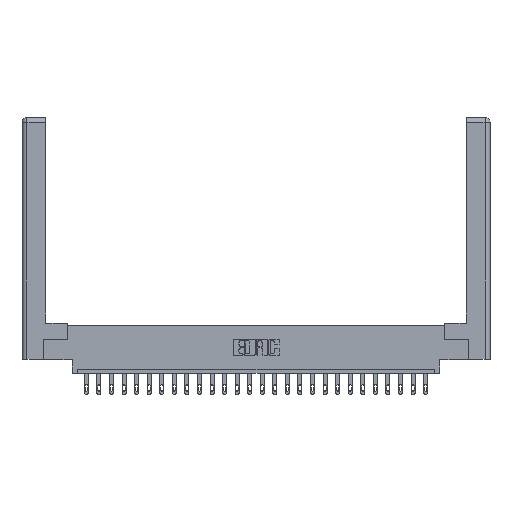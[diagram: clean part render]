
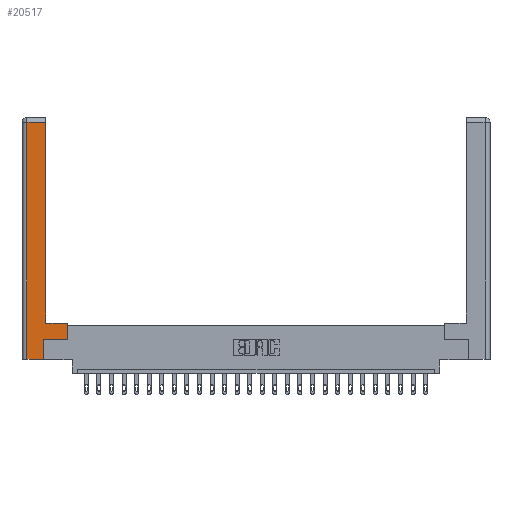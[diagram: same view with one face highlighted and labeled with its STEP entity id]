
A CAD part, top view. The second image highlights one B-rep face of the part: STEP entity #20517.
In plain terms, the highlighted planar face has unit normal (0, 0, 1).
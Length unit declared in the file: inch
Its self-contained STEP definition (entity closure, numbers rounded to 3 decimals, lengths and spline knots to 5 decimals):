
#212 = DIRECTION ( 'NONE',  ( 0., 1., 0. ) ) ;
#317 = VECTOR ( 'NONE', #12302, 39.37008 ) ;
#803 = CARTESIAN_POINT ( 'NONE',  ( 0.0615, 2.94, 0. ) ) ;
#1140 = CARTESIAN_POINT ( 'NONE',  ( 0.0615, 0., 0. ) ) ;
#1840 = CARTESIAN_POINT ( 'NONE',  ( 0.565, 0.245, 0. ) ) ;
#2126 = DIRECTION ( 'NONE',  ( -1., 0., 0. ) ) ;
#2163 = CARTESIAN_POINT ( 'NONE',  ( 0.295, 2.94, 0. ) ) ;
#2309 = ORIENTED_EDGE ( 'NONE', *, *, #22836, .T. ) ;
#2355 = CARTESIAN_POINT ( 'NONE',  ( 0.295, 0.45, 0. ) ) ;
#2630 = VECTOR ( 'NONE', #5573, 39.37008 ) ;
#3121 = ORIENTED_EDGE ( 'NONE', *, *, #6932, .T. ) ;
#3186 = ORIENTED_EDGE ( 'NONE', *, *, #24485, .T. ) ;
#3775 = CARTESIAN_POINT ( 'NONE',  ( 0.0615, 2.94, 0. ) ) ;
#4020 = ORIENTED_EDGE ( 'NONE', *, *, #15495, .T. ) ;
#4093 = VERTEX_POINT ( 'NONE', #1840 ) ;
#4378 = CARTESIAN_POINT ( 'NONE',  ( 0.295, 0.45, 0. ) ) ;
#4829 = VERTEX_POINT ( 'NONE', #2163 ) ;
#4913 = EDGE_CURVE ( 'NONE', #11134, #15058, #12675, .T. ) ;
#5312 = EDGE_CURVE ( 'NONE', #4093, #13347, #23640, .T. ) ;
#5573 = DIRECTION ( 'NONE',  ( 1., 0., 0. ) ) ;
#5865 = AXIS2_PLACEMENT_3D ( 'NONE', #18293, #6524, #23689 ) ;
#5906 = VECTOR ( 'NONE', #212, 39.37008 ) ;
#6524 = DIRECTION ( 'NONE',  ( 0., 0., -1. ) ) ;
#6556 = VECTOR ( 'NONE', #11963, 39.37008 ) ;
#6768 = VECTOR ( 'NONE', #14178, 39.37008 ) ;
#6932 = EDGE_CURVE ( 'NONE', #7507, #4093, #24185, .T. ) ;
#7394 = ORIENTED_EDGE ( 'NONE', *, *, #7652, .T. ) ;
#7507 = VERTEX_POINT ( 'NONE', #17565 ) ;
#7652 = EDGE_CURVE ( 'NONE', #17378, #7507, #19934, .T. ) ;
#7680 = VECTOR ( 'NONE', #2126, 39.37008 ) ;
#7844 = CARTESIAN_POINT ( 'NONE',  ( 0.0615, 0., 0. ) ) ;
#7941 = ORIENTED_EDGE ( 'NONE', *, *, #5312, .T. ) ;
#9828 = CARTESIAN_POINT ( 'NONE',  ( 0.295, 3., 0. ) ) ;
#11134 = VERTEX_POINT ( 'NONE', #803 ) ;
#11750 = LINE ( 'NONE', #2355, #6556 ) ;
#11867 = FACE_OUTER_BOUND ( 'NONE', #20392, .T. ) ;
#11963 = DIRECTION ( 'NONE',  ( -1., 0., 0. ) ) ;
#11996 = ORIENTED_EDGE ( 'NONE', *, *, #21440, .T. ) ;
#12302 = DIRECTION ( 'NONE',  ( 0., 1., 0. ) ) ;
#12675 = LINE ( 'NONE', #1140, #19402 ) ;
#12899 = LINE ( 'NONE', #3775, #7680 ) ;
#13347 = VERTEX_POINT ( 'NONE', #19667 ) ;
#14178 = DIRECTION ( 'NONE',  ( 1., 0., 0. ) ) ;
#14188 = PLANE ( 'NONE',  #5865 ) ;
#15058 = VERTEX_POINT ( 'NONE', #7844 ) ;
#15195 = VERTEX_POINT ( 'NONE', #4378 ) ;
#15319 = CARTESIAN_POINT ( 'NONE',  ( 0.265, 0., 0. ) ) ;
#15495 = EDGE_CURVE ( 'NONE', #13347, #15195, #11750, .T. ) ;
#15695 = CARTESIAN_POINT ( 'NONE',  ( 0.565, 0.245, 0. ) ) ;
#16761 = CARTESIAN_POINT ( 'NONE',  ( 0.265, 0., 0. ) ) ;
#17378 = VERTEX_POINT ( 'NONE', #15319 ) ;
#17565 = CARTESIAN_POINT ( 'NONE',  ( 0.265, 0.245, 0. ) ) ;
#18293 = CARTESIAN_POINT ( 'NONE',  ( 0., 0., 0. ) ) ;
#19402 = VECTOR ( 'NONE', #24981, 39.37008 ) ;
#19667 = CARTESIAN_POINT ( 'NONE',  ( 0.565, 0.45, 0. ) ) ;
#19934 = LINE ( 'NONE', #20092, #317 ) ;
#20038 = LINE ( 'NONE', #9828, #5906 ) ;
#20092 = CARTESIAN_POINT ( 'NONE',  ( 0.265, 0.245, 0. ) ) ;
#20392 = EDGE_LOOP ( 'NONE', ( #2309, #3186, #23152, #11996, #7394, #3121, #7941, #4020 ) ) ;
#20517 = ADVANCED_FACE ( 'NONE', ( #11867 ), #14188, .F. ) ;
#20714 = LINE ( 'NONE', #16761, #2630 ) ;
#20934 = VECTOR ( 'NONE', #24129, 39.37008 ) ;
#21440 = EDGE_CURVE ( 'NONE', #15058, #17378, #20714, .T. ) ;
#22274 = CARTESIAN_POINT ( 'NONE',  ( 0.565, 0.45, 0. ) ) ;
#22836 = EDGE_CURVE ( 'NONE', #15195, #4829, #20038, .T. ) ;
#23152 = ORIENTED_EDGE ( 'NONE', *, *, #4913, .T. ) ;
#23640 = LINE ( 'NONE', #22274, #20934 ) ;
#23689 = DIRECTION ( 'NONE',  ( -1., 0., 0. ) ) ;
#24129 = DIRECTION ( 'NONE',  ( 0., 1., 0. ) ) ;
#24185 = LINE ( 'NONE', #15695, #6768 ) ;
#24485 = EDGE_CURVE ( 'NONE', #4829, #11134, #12899, .T. ) ;
#24981 = DIRECTION ( 'NONE',  ( 0., -1., 0. ) ) ;
